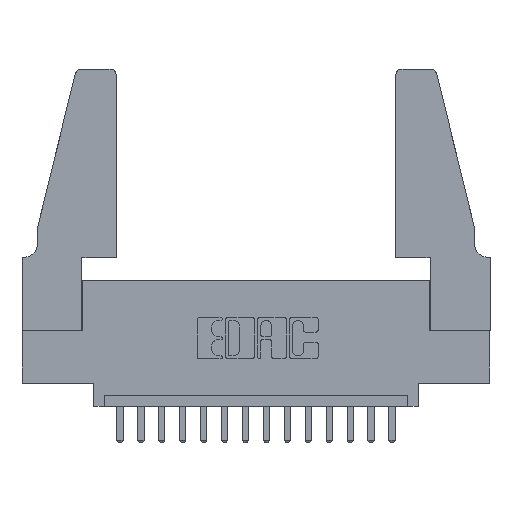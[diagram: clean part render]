
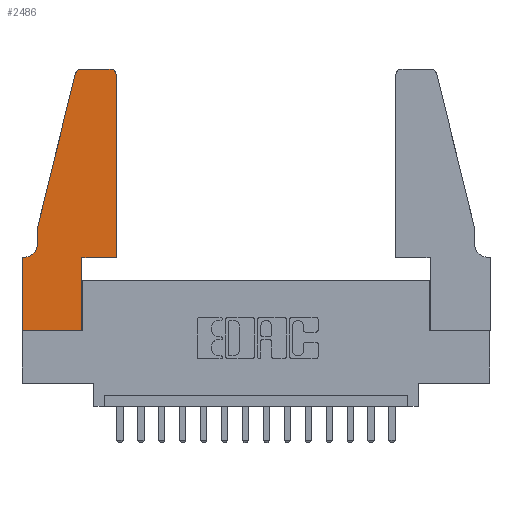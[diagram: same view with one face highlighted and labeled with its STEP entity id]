
A CAD part, top view. The second image highlights one B-rep face of the part: STEP entity #2486.
In plain terms, the highlighted planar face has unit normal (0, 0, 1).
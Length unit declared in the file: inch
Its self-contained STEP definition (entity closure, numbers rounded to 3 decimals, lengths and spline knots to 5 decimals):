
#33 = DIRECTION ( 'NONE',  ( -0.239, -0.971, 0. ) ) ;
#35 = LINE ( 'NONE', #3422, #13413 ) ;
#351 = LINE ( 'NONE', #1832, #6846 ) ;
#475 = DIRECTION ( 'NONE',  ( 0., 0., -1. ) ) ;
#521 = DIRECTION ( 'NONE',  ( 0., 0., 1. ) ) ;
#581 = AXIS2_PLACEMENT_3D ( 'NONE', #4662, #12435, #14943 ) ;
#587 = DIRECTION ( 'NONE',  ( -1., 0., 0. ) ) ;
#985 = PLANE ( 'NONE',  #8386 ) ;
#1497 = AXIS2_PLACEMENT_3D ( 'NONE', #5767, #521, #14706 ) ;
#1832 = CARTESIAN_POINT ( 'NONE',  ( 0.0755, 0.35, 0.37 ) ) ;
#2077 = DIRECTION ( 'NONE',  ( 1., 0., 0. ) ) ;
#2365 = AXIS2_PLACEMENT_3D ( 'NONE', #3330, #475, #587 ) ;
#2445 = EDGE_CURVE ( 'NONE', #6143, #5519, #12708, .T. ) ;
#2486 = ADVANCED_FACE ( 'NONE', ( #7055 ), #985, .T. ) ;
#2536 = CARTESIAN_POINT ( 'NONE',  ( 0.4505, 0.35, 0.37 ) ) ;
#2597 = VERTEX_POINT ( 'NONE', #4910 ) ;
#2663 = VECTOR ( 'NONE', #12813, 39.37008 ) ;
#2674 = VERTEX_POINT ( 'NONE', #16648 ) ;
#2756 = DIRECTION ( 'NONE',  ( 0., -1., 0. ) ) ;
#2766 = CARTESIAN_POINT ( 'NONE',  ( 0.4505, 0.35, 0.37 ) ) ;
#3095 = CARTESIAN_POINT ( 'NONE',  ( 0.0755, 0.5, 0.37 ) ) ;
#3212 = ORIENTED_EDGE ( 'NONE', *, *, #8011, .T. ) ;
#3330 = CARTESIAN_POINT ( 'NONE',  ( 0.0055, 0.42, 0.37 ) ) ;
#3422 = CARTESIAN_POINT ( 'NONE',  ( 0.0755, 0.5, 0.37 ) ) ;
#4019 = LINE ( 'NONE', #2536, #6637 ) ;
#4101 = DIRECTION ( 'NONE',  ( 0., 1., 0. ) ) ;
#4230 = VERTEX_POINT ( 'NONE', #16114 ) ;
#4316 = CARTESIAN_POINT ( 'NONE',  ( 0.2865, 0.35, 0.37 ) ) ;
#4662 = CARTESIAN_POINT ( 'NONE',  ( 0.4205, 1.22, 0.37 ) ) ;
#4910 = CARTESIAN_POINT ( 'NONE',  ( 0., 0.35, 0.37 ) ) ;
#5050 = VERTEX_POINT ( 'NONE', #14266 ) ;
#5205 = ORIENTED_EDGE ( 'NONE', *, *, #16228, .T. ) ;
#5485 = CARTESIAN_POINT ( 'NONE',  ( 0.0755, 0.42, 0.37 ) ) ;
#5519 = VERTEX_POINT ( 'NONE', #14419 ) ;
#5667 = VECTOR ( 'NONE', #33, 39.37008 ) ;
#5767 = CARTESIAN_POINT ( 'NONE',  ( 0.284, 1.22, 0.37 ) ) ;
#6081 = EDGE_CURVE ( 'NONE', #11496, #6464, #9181, .T. ) ;
#6143 = VERTEX_POINT ( 'NONE', #10417 ) ;
#6250 = VECTOR ( 'NONE', #4101, 39.37008 ) ;
#6464 = VERTEX_POINT ( 'NONE', #7362 ) ;
#6637 = VECTOR ( 'NONE', #8923, 39.37008 ) ;
#6803 = ORIENTED_EDGE ( 'NONE', *, *, #2445, .T. ) ;
#6846 = VECTOR ( 'NONE', #8427, 39.37008 ) ;
#6926 = ORIENTED_EDGE ( 'NONE', *, *, #9939, .T. ) ;
#7055 = FACE_OUTER_BOUND ( 'NONE', #12806, .T. ) ;
#7286 = LINE ( 'NONE', #11755, #14338 ) ;
#7362 = CARTESIAN_POINT ( 'NONE',  ( 0.0055, 0.35, 0.37 ) ) ;
#8007 = ORIENTED_EDGE ( 'NONE', *, *, #13754, .T. ) ;
#8011 = EDGE_CURVE ( 'NONE', #6464, #2597, #351, .T. ) ;
#8262 = VECTOR ( 'NONE', #13598, 39.37008 ) ;
#8386 = AXIS2_PLACEMENT_3D ( 'NONE', #9800, #9963, #2077 ) ;
#8427 = DIRECTION ( 'NONE',  ( -1., 0., 0. ) ) ;
#8659 = DIRECTION ( 'NONE',  ( 0., -1., 0. ) ) ;
#8923 = DIRECTION ( 'NONE',  ( 1., 0., 0. ) ) ;
#8930 = LINE ( 'NONE', #2766, #2663 ) ;
#9070 = LINE ( 'NONE', #10414, #5667 ) ;
#9181 = CIRCLE ( 'NONE', #2365, 0.07 ) ;
#9225 = LINE ( 'NONE', #15692, #11449 ) ;
#9800 = CARTESIAN_POINT ( 'NONE',  ( 0., 0.35, 0.37 ) ) ;
#9939 = EDGE_CURVE ( 'NONE', #11638, #11496, #35, .T. ) ;
#9963 = DIRECTION ( 'NONE',  ( 0., 0., 1. ) ) ;
#10414 = CARTESIAN_POINT ( 'NONE',  ( 0.0755, 0.5, 0.37 ) ) ;
#10417 = CARTESIAN_POINT ( 'NONE',  ( 0., 0., 0.37 ) ) ;
#10514 = CIRCLE ( 'NONE', #581, 0.03 ) ;
#10822 = CARTESIAN_POINT ( 'NONE',  ( 0.25487, 1.22718, 0.37 ) ) ;
#10830 = ORIENTED_EDGE ( 'NONE', *, *, #15817, .T. ) ;
#11031 = ORIENTED_EDGE ( 'NONE', *, *, #11310, .T. ) ;
#11059 = CARTESIAN_POINT ( 'NONE',  ( 0., 0., 0.37 ) ) ;
#11310 = EDGE_CURVE ( 'NONE', #2674, #14655, #8930, .T. ) ;
#11449 = VECTOR ( 'NONE', #2756, 39.37008 ) ;
#11496 = VERTEX_POINT ( 'NONE', #5485 ) ;
#11638 = VERTEX_POINT ( 'NONE', #3095 ) ;
#11755 = CARTESIAN_POINT ( 'NONE',  ( 0.2605, 1.25, 0.37 ) ) ;
#11901 = LINE ( 'NONE', #4316, #6250 ) ;
#12435 = DIRECTION ( 'NONE',  ( 0., 0., 1. ) ) ;
#12708 = LINE ( 'NONE', #11059, #8262 ) ;
#12713 = VERTEX_POINT ( 'NONE', #15582 ) ;
#12806 = EDGE_LOOP ( 'NONE', ( #8007, #5205, #15884, #6926, #16177, #3212, #15041, #6803, #16429, #10830, #11031, #13032 ) ) ;
#12813 = DIRECTION ( 'NONE',  ( 0., 1., 0. ) ) ;
#12970 = EDGE_CURVE ( 'NONE', #14655, #4230, #10514, .T. ) ;
#13032 = ORIENTED_EDGE ( 'NONE', *, *, #12970, .T. ) ;
#13413 = VECTOR ( 'NONE', #8659, 39.37008 ) ;
#13598 = DIRECTION ( 'NONE',  ( 1., 0., 0. ) ) ;
#13628 = CARTESIAN_POINT ( 'NONE',  ( 0.4505, 1.22, 0.37 ) ) ;
#13754 = EDGE_CURVE ( 'NONE', #4230, #12713, #7286, .T. ) ;
#14266 = CARTESIAN_POINT ( 'NONE',  ( 0.2865, 0.35, 0.37 ) ) ;
#14338 = VECTOR ( 'NONE', #15550, 39.37008 ) ;
#14419 = CARTESIAN_POINT ( 'NONE',  ( 0.2865, 0., 0.37 ) ) ;
#14629 = VERTEX_POINT ( 'NONE', #10822 ) ;
#14655 = VERTEX_POINT ( 'NONE', #13628 ) ;
#14706 = DIRECTION ( 'NONE',  ( 1., 0., 0. ) ) ;
#14943 = DIRECTION ( 'NONE',  ( 1., 0., 0. ) ) ;
#15041 = ORIENTED_EDGE ( 'NONE', *, *, #16669, .T. ) ;
#15210 = EDGE_CURVE ( 'NONE', #14629, #11638, #9070, .T. ) ;
#15379 = EDGE_CURVE ( 'NONE', #5519, #5050, #11901, .T. ) ;
#15550 = DIRECTION ( 'NONE',  ( -1., 0., 0. ) ) ;
#15582 = CARTESIAN_POINT ( 'NONE',  ( 0.284, 1.25, 0.37 ) ) ;
#15692 = CARTESIAN_POINT ( 'NONE',  ( 0., 0., 0.37 ) ) ;
#15817 = EDGE_CURVE ( 'NONE', #5050, #2674, #4019, .T. ) ;
#15868 = CIRCLE ( 'NONE', #1497, 0.03 ) ;
#15884 = ORIENTED_EDGE ( 'NONE', *, *, #15210, .T. ) ;
#16114 = CARTESIAN_POINT ( 'NONE',  ( 0.4205, 1.25, 0.37 ) ) ;
#16177 = ORIENTED_EDGE ( 'NONE', *, *, #6081, .T. ) ;
#16228 = EDGE_CURVE ( 'NONE', #12713, #14629, #15868, .T. ) ;
#16429 = ORIENTED_EDGE ( 'NONE', *, *, #15379, .T. ) ;
#16648 = CARTESIAN_POINT ( 'NONE',  ( 0.4505, 0.35, 0.37 ) ) ;
#16669 = EDGE_CURVE ( 'NONE', #2597, #6143, #9225, .T. ) ;
